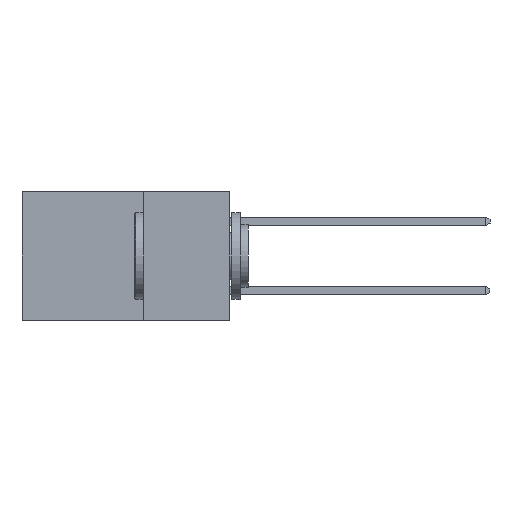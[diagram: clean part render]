
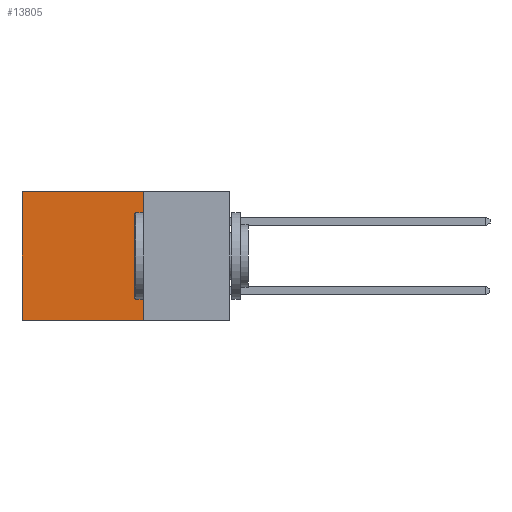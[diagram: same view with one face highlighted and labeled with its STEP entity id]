
A CAD part, left-side view. The second image highlights one B-rep face of the part: STEP entity #13805.
In plain terms, the highlighted planar face has unit normal (-1, 0, 0).
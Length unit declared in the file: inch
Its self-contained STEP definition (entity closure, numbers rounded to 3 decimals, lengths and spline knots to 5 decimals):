
#108 = DIRECTION ( 'NONE',  ( 0., 1., 0. ) ) ;
#907 = AXIS2_PLACEMENT_3D ( 'NONE', #14497, #5045, #16084 ) ;
#988 = LINE ( 'NONE', #18234, #17739 ) ;
#1409 = EDGE_LOOP ( 'NONE', ( #1998, #6357, #1691, #7264 ) ) ;
#1419 = CARTESIAN_POINT ( 'NONE',  ( 0.298, 0.6, 0. ) ) ;
#1519 = EDGE_CURVE ( 'NONE', #10033, #19083, #1686, .T. ) ;
#1686 = LINE ( 'NONE', #4157, #18447 ) ;
#1691 = ORIENTED_EDGE ( 'NONE', *, *, #4673, .F. ) ;
#1998 = ORIENTED_EDGE ( 'NONE', *, *, #12746, .T. ) ;
#2342 = CARTESIAN_POINT ( 'NONE',  ( 0.298, 0.25, -0.37 ) ) ;
#3237 = LINE ( 'NONE', #13781, #6938 ) ;
#4157 = CARTESIAN_POINT ( 'NONE',  ( 0.298, 0.25, 0. ) ) ;
#4673 = EDGE_CURVE ( 'NONE', #10033, #20275, #16645, .T. ) ;
#5045 = DIRECTION ( 'NONE',  ( 1., 0., 0. ) ) ;
#6357 = ORIENTED_EDGE ( 'NONE', *, *, #16964, .F. ) ;
#6938 = VECTOR ( 'NONE', #15381, 39.37008 ) ;
#7264 = ORIENTED_EDGE ( 'NONE', *, *, #1519, .T. ) ;
#8791 = DIRECTION ( 'NONE',  ( 0., 0., -1. ) ) ;
#10033 = VERTEX_POINT ( 'NONE', #14537 ) ;
#11305 = PLANE ( 'NONE',  #907 ) ;
#11558 = VERTEX_POINT ( 'NONE', #15052 ) ;
#11942 = VECTOR ( 'NONE', #19520, 39.37008 ) ;
#12746 = EDGE_CURVE ( 'NONE', #19083, #11558, #988, .T. ) ;
#13781 = CARTESIAN_POINT ( 'NONE',  ( 0.298, 0.25, -0.37 ) ) ;
#13805 = ADVANCED_FACE ( 'NONE', ( #18632 ), #11305, .F. ) ;
#14497 = CARTESIAN_POINT ( 'NONE',  ( 0.298, 0.25, 0. ) ) ;
#14537 = CARTESIAN_POINT ( 'NONE',  ( 0.298, 0.25, 0. ) ) ;
#15052 = CARTESIAN_POINT ( 'NONE',  ( 0.298, 0.6, -0.37 ) ) ;
#15381 = DIRECTION ( 'NONE',  ( 0., 1., 0. ) ) ;
#16084 = DIRECTION ( 'NONE',  ( 0., 0., -1. ) ) ;
#16645 = LINE ( 'NONE', #18040, #11942 ) ;
#16964 = EDGE_CURVE ( 'NONE', #20275, #11558, #3237, .T. ) ;
#17739 = VECTOR ( 'NONE', #8791, 39.37008 ) ;
#18040 = CARTESIAN_POINT ( 'NONE',  ( 0.298, 0.25, 0. ) ) ;
#18234 = CARTESIAN_POINT ( 'NONE',  ( 0.298, 0.6, 0. ) ) ;
#18447 = VECTOR ( 'NONE', #108, 39.37008 ) ;
#18632 = FACE_OUTER_BOUND ( 'NONE', #1409, .T. ) ;
#19083 = VERTEX_POINT ( 'NONE', #1419 ) ;
#19520 = DIRECTION ( 'NONE',  ( 0., 0., -1. ) ) ;
#20275 = VERTEX_POINT ( 'NONE', #2342 ) ;
